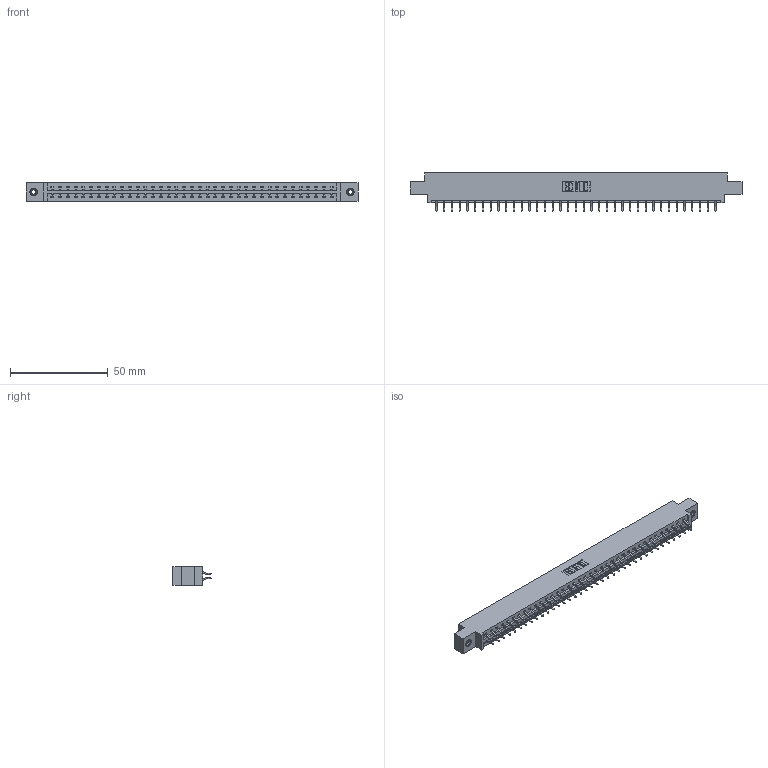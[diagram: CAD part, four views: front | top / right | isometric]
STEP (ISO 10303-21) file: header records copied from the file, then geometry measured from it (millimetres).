
FILE_DESCRIPTION (( 'STEP AP203' ), '1' );
FILE_NAME ('387-074-556-808.STEP', '2018-09-22T20:27:38', ( '' ), ( '' ), 'SwSTEP 2.0', 'SolidWorks 2016', '' );
FILE_SCHEMA (( 'CONFIG_CONTROL_DESIGN' ));
Length unit declared in the file: inch
Products named in the file (4): 337 Part_0.170 Offset - 0.156 Dia-TI; 345-292-001_556 Tail; 345-250-001_345-250-003-102; 387-074-556-808
Assembly tree (77 placements, depth 2):
  387-074-556-808
    337 Part_0.170 Offset - 0.156 Dia-TI
    345-292-001_556 Tail  x74
    345-250-001_345-250-003-102  x2
Bounding box: 169.62 x 19.57 x 9.4 mm (x, y, z)
Volume: 17682.5 mm3; surface area: 19995.2 mm2
Topology: 77 solids, 77 shells, 4618 faces, 13705 edges, 9030 vertices
Faces by surface type: plane 3214, cylinder 1388, cone 12, torus 4
Entity records: 30872 total; most frequent: CARTESIAN_POINT 5201, ORIENTED_EDGE 5118, DIRECTION 4453, EDGE_CURVE 2559, LINE 2403, VECTOR 2403, VERTEX_POINT 1700, AXIS2_PLACEMENT_3D 1025
